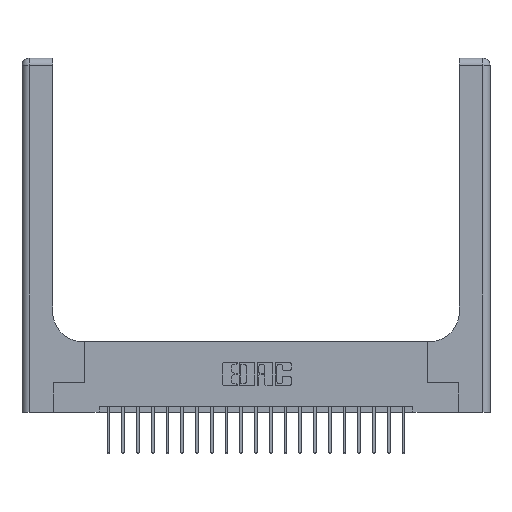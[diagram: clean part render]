
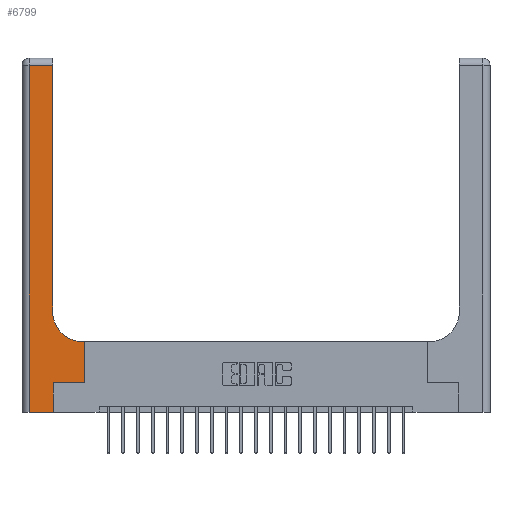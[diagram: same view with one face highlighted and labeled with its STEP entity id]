
A CAD part, top view. The second image highlights one B-rep face of the part: STEP entity #6799.
In plain terms, the highlighted planar face has unit normal (0, 0, 1).
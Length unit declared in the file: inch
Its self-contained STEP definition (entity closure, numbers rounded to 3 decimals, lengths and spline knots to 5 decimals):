
#188 = CARTESIAN_POINT ( 'NONE',  ( 0.528, 0.25, 0.37 ) ) ;
#927 = DIRECTION ( 'NONE',  ( 0., 0., -1. ) ) ;
#1260 = VERTEX_POINT ( 'NONE', #20972 ) ;
#1475 = AXIS2_PLACEMENT_3D ( 'NONE', #2212, #19012, #7263 ) ;
#1859 = VERTEX_POINT ( 'NONE', #16813 ) ;
#1905 = ORIENTED_EDGE ( 'NONE', *, *, #10307, .T. ) ;
#1918 = LINE ( 'NONE', #13031, #10557 ) ;
#2065 = ORIENTED_EDGE ( 'NONE', *, *, #15331, .T. ) ;
#2154 = DIRECTION ( 'NONE',  ( 0., 1., 0. ) ) ;
#2212 = CARTESIAN_POINT ( 'NONE',  ( 0., 3., 0.37 ) ) ;
#2334 = VECTOR ( 'NONE', #17575, 39.37008 ) ;
#2405 = VECTOR ( 'NONE', #7166, 39.37008 ) ;
#2765 = FACE_OUTER_BOUND ( 'NONE', #14359, .T. ) ;
#2877 = LINE ( 'NONE', #10962, #2334 ) ;
#3005 = ORIENTED_EDGE ( 'NONE', *, *, #13723, .T. ) ;
#3030 = EDGE_CURVE ( 'NONE', #16991, #4404, #4250, .T. ) ;
#3341 = DIRECTION ( 'NONE',  ( 0., -1., 0. ) ) ;
#4153 = LINE ( 'NONE', #9794, #6505 ) ;
#4224 = DIRECTION ( 'NONE',  ( 1., 0., 0. ) ) ;
#4250 = LINE ( 'NONE', #16397, #16050 ) ;
#4295 = ORIENTED_EDGE ( 'NONE', *, *, #19544, .T. ) ;
#4404 = VERTEX_POINT ( 'NONE', #188 ) ;
#4417 = ORIENTED_EDGE ( 'NONE', *, *, #8531, .T. ) ;
#4628 = ORIENTED_EDGE ( 'NONE', *, *, #11605, .T. ) ;
#4629 = LINE ( 'NONE', #17041, #16159 ) ;
#5288 = CARTESIAN_POINT ( 'NONE',  ( 0.51, 0.6, 0.37 ) ) ;
#5536 = VERTEX_POINT ( 'NONE', #6898 ) ;
#5747 = CARTESIAN_POINT ( 'NONE',  ( 0.26, 0.85, 0.37 ) ) ;
#6336 = DIRECTION ( 'NONE',  ( 1., 0., 0. ) ) ;
#6350 = LINE ( 'NONE', #20755, #19505 ) ;
#6505 = VECTOR ( 'NONE', #14942, 39.37008 ) ;
#6799 = ADVANCED_FACE ( 'NONE', ( #2765 ), #20635, .F. ) ;
#6898 = CARTESIAN_POINT ( 'NONE',  ( 0.26, 2.94, 0.37 ) ) ;
#7166 = DIRECTION ( 'NONE',  ( -1., 0., 0. ) ) ;
#7263 = DIRECTION ( 'NONE',  ( -1., 0., 0. ) ) ;
#7694 = CARTESIAN_POINT ( 'NONE',  ( 0.06, 0., 0.37 ) ) ;
#8107 = VERTEX_POINT ( 'NONE', #7694 ) ;
#8531 = EDGE_CURVE ( 'NONE', #8107, #1260, #6350, .T. ) ;
#8743 = VERTEX_POINT ( 'NONE', #11357 ) ;
#8857 = ORIENTED_EDGE ( 'NONE', *, *, #13469, .T. ) ;
#8992 = LINE ( 'NONE', #10649, #21622 ) ;
#9676 = ORIENTED_EDGE ( 'NONE', *, *, #3030, .T. ) ;
#9794 = CARTESIAN_POINT ( 'NONE',  ( 0.528, 0.25, 0.37 ) ) ;
#10278 = VERTEX_POINT ( 'NONE', #5747 ) ;
#10307 = EDGE_CURVE ( 'NONE', #5536, #8743, #2877, .T. ) ;
#10557 = VECTOR ( 'NONE', #3341, 39.37008 ) ;
#10649 = CARTESIAN_POINT ( 'NONE',  ( 0.26, 3., 0.37 ) ) ;
#10682 = DIRECTION ( 'NONE',  ( 1., 0., 0. ) ) ;
#10962 = CARTESIAN_POINT ( 'NONE',  ( 0., 2.94, 0.37 ) ) ;
#11357 = CARTESIAN_POINT ( 'NONE',  ( 0.06, 2.94, 0.37 ) ) ;
#11536 = CARTESIAN_POINT ( 'NONE',  ( 0.265, 0.25, 0.37 ) ) ;
#11537 = AXIS2_PLACEMENT_3D ( 'NONE', #14208, #927, #4224 ) ;
#11605 = EDGE_CURVE ( 'NONE', #4404, #1859, #4153, .T. ) ;
#11816 = CARTESIAN_POINT ( 'NONE',  ( 0.26, 0.6, 0.37 ) ) ;
#13031 = CARTESIAN_POINT ( 'NONE',  ( 0.06, 3., 0.37 ) ) ;
#13469 = EDGE_CURVE ( 'NONE', #10278, #5536, #8992, .T. ) ;
#13723 = EDGE_CURVE ( 'NONE', #17759, #10278, #21081, .T. ) ;
#13854 = EDGE_CURVE ( 'NONE', #8743, #8107, #1918, .T. ) ;
#14208 = CARTESIAN_POINT ( 'NONE',  ( 0.51, 0.85, 0.37 ) ) ;
#14359 = EDGE_LOOP ( 'NONE', ( #8857, #1905, #16059, #4417, #4295, #9676, #4628, #2065, #3005 ) ) ;
#14942 = DIRECTION ( 'NONE',  ( 0., 1., 0. ) ) ;
#15331 = EDGE_CURVE ( 'NONE', #1859, #17759, #15773, .T. ) ;
#15608 = DIRECTION ( 'NONE',  ( 0., 1., 0. ) ) ;
#15773 = LINE ( 'NONE', #11816, #2405 ) ;
#16050 = VECTOR ( 'NONE', #6336, 39.37008 ) ;
#16059 = ORIENTED_EDGE ( 'NONE', *, *, #13854, .T. ) ;
#16159 = VECTOR ( 'NONE', #15608, 39.37008 ) ;
#16397 = CARTESIAN_POINT ( 'NONE',  ( 0.265, 0.25, 0.37 ) ) ;
#16813 = CARTESIAN_POINT ( 'NONE',  ( 0.528, 0.6, 0.37 ) ) ;
#16991 = VERTEX_POINT ( 'NONE', #11536 ) ;
#17041 = CARTESIAN_POINT ( 'NONE',  ( 0.265, 0., 0.37 ) ) ;
#17575 = DIRECTION ( 'NONE',  ( -1., 0., 0. ) ) ;
#17759 = VERTEX_POINT ( 'NONE', #5288 ) ;
#19012 = DIRECTION ( 'NONE',  ( 0., 0., -1. ) ) ;
#19505 = VECTOR ( 'NONE', #10682, 39.37008 ) ;
#19544 = EDGE_CURVE ( 'NONE', #1260, #16991, #4629, .T. ) ;
#20635 = PLANE ( 'NONE',  #1475 ) ;
#20755 = CARTESIAN_POINT ( 'NONE',  ( 0., 0., 0.37 ) ) ;
#20972 = CARTESIAN_POINT ( 'NONE',  ( 0.265, 0., 0.37 ) ) ;
#21081 = CIRCLE ( 'NONE', #11537, 0.25 ) ;
#21622 = VECTOR ( 'NONE', #2154, 39.37008 ) ;
